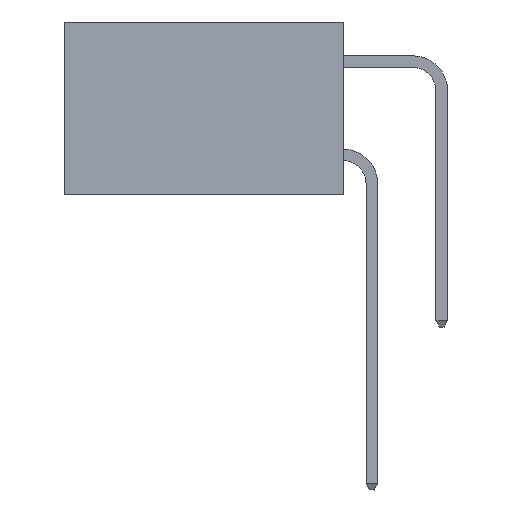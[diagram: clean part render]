
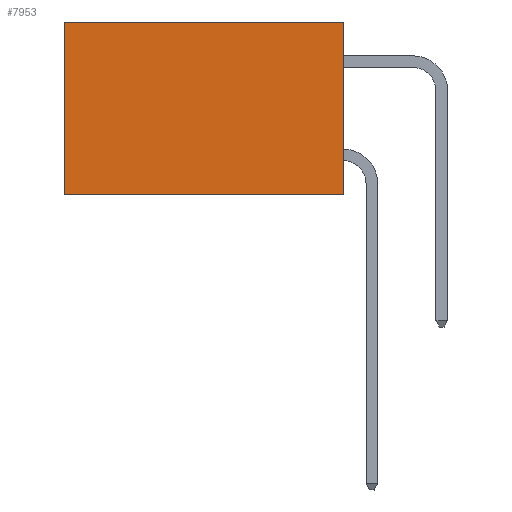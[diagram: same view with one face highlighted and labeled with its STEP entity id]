
A CAD part, left-side view. The second image highlights one B-rep face of the part: STEP entity #7953.
In plain terms, the highlighted planar face has unit normal (-1, 0, 0).
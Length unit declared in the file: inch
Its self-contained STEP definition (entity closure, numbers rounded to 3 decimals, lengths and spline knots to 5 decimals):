
#1286 = CARTESIAN_POINT ( 'NONE',  ( 0.2615, 0., -0.37 ) ) ;
#1951 = AXIS2_PLACEMENT_3D ( 'NONE', #9410, #2080, #10607 ) ;
#1983 = PLANE ( 'NONE',  #1951 ) ;
#2002 = EDGE_LOOP ( 'NONE', ( #8411, #11569, #15065, #5859 ) ) ;
#2057 = DIRECTION ( 'NONE',  ( 0., 1., 0. ) ) ;
#2080 = DIRECTION ( 'NONE',  ( 1., 0., 0. ) ) ;
#3547 = FACE_OUTER_BOUND ( 'NONE', #2002, .T. ) ;
#3621 = CARTESIAN_POINT ( 'NONE',  ( 0.2615, 0., -0.37 ) ) ;
#5039 = EDGE_CURVE ( 'NONE', #5405, #14852, #5775, .T. ) ;
#5318 = EDGE_CURVE ( 'NONE', #10451, #5405, #9586, .T. ) ;
#5405 = VERTEX_POINT ( 'NONE', #14764 ) ;
#5705 = LINE ( 'NONE', #7387, #11828 ) ;
#5775 = LINE ( 'NONE', #8917, #7423 ) ;
#5859 = ORIENTED_EDGE ( 'NONE', *, *, #5318, .T. ) ;
#6900 = CARTESIAN_POINT ( 'NONE',  ( 0.2615, 0.6, -0.37 ) ) ;
#7387 = CARTESIAN_POINT ( 'NONE',  ( 0.2615, 0., -0.37 ) ) ;
#7423 = VECTOR ( 'NONE', #14889, 39.37008 ) ;
#7953 = ADVANCED_FACE ( 'NONE', ( #3547 ), #1983, .F. ) ;
#8411 = ORIENTED_EDGE ( 'NONE', *, *, #5039, .T. ) ;
#8618 = LINE ( 'NONE', #1286, #17746 ) ;
#8753 = DIRECTION ( 'NONE',  ( 0., 1., 0. ) ) ;
#8917 = CARTESIAN_POINT ( 'NONE',  ( 0.2615, 0.6, -0.37 ) ) ;
#9410 = CARTESIAN_POINT ( 'NONE',  ( 0.2615, 0., -0.37 ) ) ;
#9586 = LINE ( 'NONE', #14284, #14275 ) ;
#10451 = VERTEX_POINT ( 'NONE', #18851 ) ;
#10607 = DIRECTION ( 'NONE',  ( 0., 0., -1. ) ) ;
#11569 = ORIENTED_EDGE ( 'NONE', *, *, #17040, .F. ) ;
#11828 = VECTOR ( 'NONE', #8753, 39.37008 ) ;
#14275 = VECTOR ( 'NONE', #2057, 39.37008 ) ;
#14284 = CARTESIAN_POINT ( 'NONE',  ( 0.2615, 0., 0. ) ) ;
#14399 = DIRECTION ( 'NONE',  ( 0., 0., -1. ) ) ;
#14764 = CARTESIAN_POINT ( 'NONE',  ( 0.2615, 0.6, 0. ) ) ;
#14852 = VERTEX_POINT ( 'NONE', #6900 ) ;
#14889 = DIRECTION ( 'NONE',  ( 0., 0., -1. ) ) ;
#15065 = ORIENTED_EDGE ( 'NONE', *, *, #16405, .F. ) ;
#15616 = VERTEX_POINT ( 'NONE', #3621 ) ;
#16405 = EDGE_CURVE ( 'NONE', #10451, #15616, #8618, .T. ) ;
#17040 = EDGE_CURVE ( 'NONE', #15616, #14852, #5705, .T. ) ;
#17746 = VECTOR ( 'NONE', #14399, 39.37008 ) ;
#18851 = CARTESIAN_POINT ( 'NONE',  ( 0.2615, 0., 0. ) ) ;
